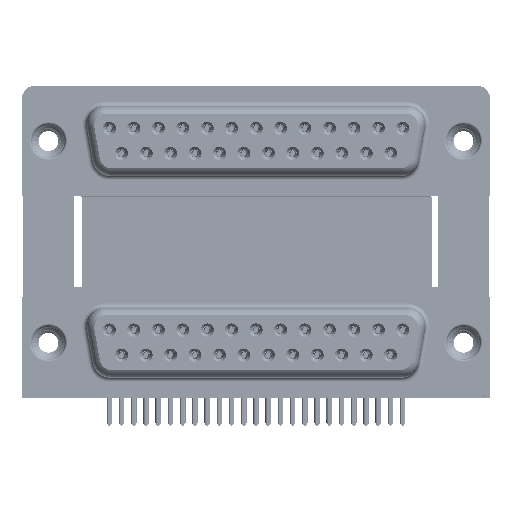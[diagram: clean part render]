
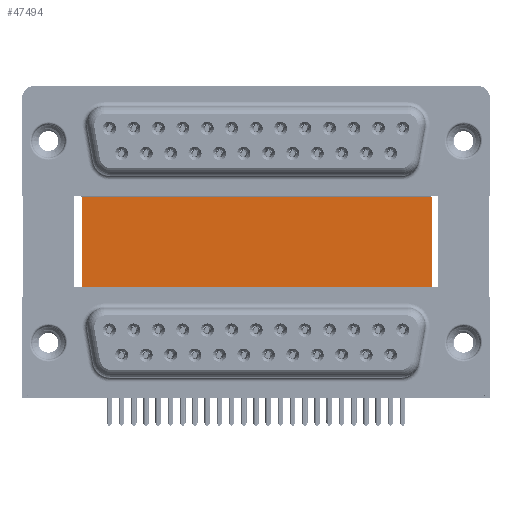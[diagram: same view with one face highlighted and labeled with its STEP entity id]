
A CAD part, top view. The second image highlights one B-rep face of the part: STEP entity #47494.
In plain terms, the highlighted planar face has unit normal (0, 0, 1).
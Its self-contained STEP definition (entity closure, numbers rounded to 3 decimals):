
#470 = LINE ( 'NONE', #19261, #15147 ) ;
#1281 = DIRECTION ( 'NONE',  ( -1., 0., 0. ) ) ;
#3389 = LINE ( 'NONE', #42488, #17976 ) ;
#5720 = VERTEX_POINT ( 'NONE', #22375 ) ;
#6290 = VECTOR ( 'NONE', #31096, 1000. ) ;
#6961 = VECTOR ( 'NONE', #21916, 1000. ) ;
#8991 = VERTEX_POINT ( 'NONE', #33069 ) ;
#11168 = DIRECTION ( 'NONE',  ( 0., 0., -1. ) ) ;
#11467 = CARTESIAN_POINT ( 'NONE',  ( 3.79, 16.585, -12. ) ) ;
#11709 = LINE ( 'NONE', #21549, #6290 ) ;
#13089 = EDGE_CURVE ( 'NONE', #8991, #5720, #60077, .T. ) ;
#13242 = ORIENTED_EDGE ( 'NONE', *, *, #14816, .F. ) ;
#13279 = ORIENTED_EDGE ( 'NONE', *, *, #13089, .F. ) ;
#14816 = EDGE_CURVE ( 'NONE', #5720, #39085, #11709, .T. ) ;
#14992 = FACE_OUTER_BOUND ( 'NONE', #45515, .T. ) ;
#15147 = VECTOR ( 'NONE', #18943, 1000. ) ;
#16828 = CARTESIAN_POINT ( 'NONE',  ( 3.79, 16.585, -12. ) ) ;
#17976 = VECTOR ( 'NONE', #41861, 1000. ) ;
#18943 = DIRECTION ( 'NONE',  ( 0., -1., 0. ) ) ;
#19261 = CARTESIAN_POINT ( 'NONE',  ( 3.79, 16.585, -12. ) ) ;
#21549 = CARTESIAN_POINT ( 'NONE',  ( 43.43, 16.585, -12. ) ) ;
#21916 = DIRECTION ( 'NONE',  ( 1., 0., 0. ) ) ;
#22375 = CARTESIAN_POINT ( 'NONE',  ( 43.43, 16.585, -12. ) ) ;
#22992 = EDGE_CURVE ( 'NONE', #8991, #39497, #470, .T. ) ;
#25163 = PLANE ( 'NONE',  #55841 ) ;
#25374 = CARTESIAN_POINT ( 'NONE',  ( 43.43, -3.735, -12. ) ) ;
#31096 = DIRECTION ( 'NONE',  ( 0., -1., 0. ) ) ;
#33069 = CARTESIAN_POINT ( 'NONE',  ( 3.79, 16.585, -12. ) ) ;
#38769 = ORIENTED_EDGE ( 'NONE', *, *, #55604, .T. ) ;
#39085 = VERTEX_POINT ( 'NONE', #25374 ) ;
#39497 = VERTEX_POINT ( 'NONE', #56412 ) ;
#41861 = DIRECTION ( 'NONE',  ( 1., 0., 0. ) ) ;
#42488 = CARTESIAN_POINT ( 'NONE',  ( 3.79, -3.735, -12. ) ) ;
#45515 = EDGE_LOOP ( 'NONE', ( #38769, #13242, #13279, #51606 ) ) ;
#47494 = ADVANCED_FACE ( 'NONE', ( #14992 ), #25163, .F. ) ;
#51606 = ORIENTED_EDGE ( 'NONE', *, *, #22992, .T. ) ;
#55604 = EDGE_CURVE ( 'NONE', #39497, #39085, #3389, .T. ) ;
#55841 = AXIS2_PLACEMENT_3D ( 'NONE', #11467, #11168, #1281 ) ;
#56412 = CARTESIAN_POINT ( 'NONE',  ( 3.79, -3.735, -12. ) ) ;
#60077 = LINE ( 'NONE', #16828, #6961 ) ;
